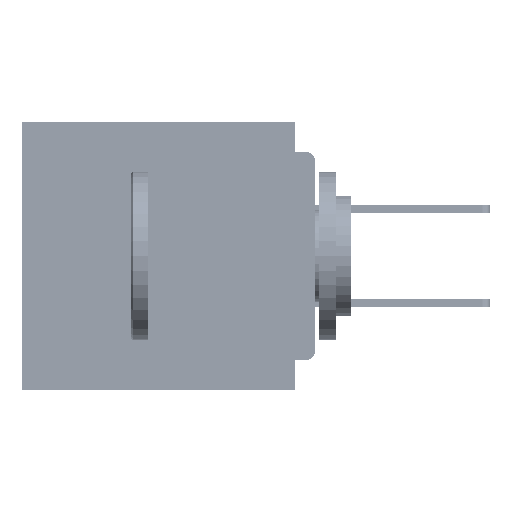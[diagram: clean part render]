
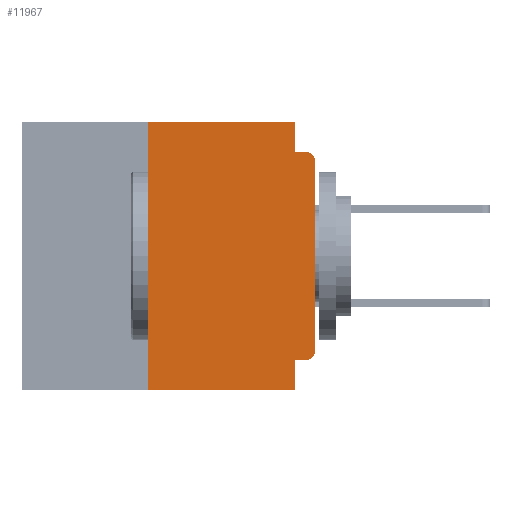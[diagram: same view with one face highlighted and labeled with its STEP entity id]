
A CAD part, left-side view. The second image highlights one B-rep face of the part: STEP entity #11967.
In plain terms, the highlighted planar face has unit normal (-1, 0, 0).
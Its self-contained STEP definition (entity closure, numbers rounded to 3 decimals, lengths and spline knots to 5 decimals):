
#201 = VERTEX_POINT ( 'NONE', #17574 ) ;
#924 = DIRECTION ( 'NONE',  ( 0., 0., -1. ) ) ;
#1513 = EDGE_LOOP ( 'NONE', ( #3939, #25985, #49332, #69862, #61887, #24744, #14929, #63071, #38766, #44028 ) ) ;
#2247 = CARTESIAN_POINT ( 'NONE',  ( 0., 0., -0.045 ) ) ;
#2637 = VERTEX_POINT ( 'NONE', #37194 ) ;
#2857 = CARTESIAN_POINT ( 'NONE',  ( 0., 0.031, -0.4 ) ) ;
#3939 = ORIENTED_EDGE ( 'NONE', *, *, #6980, .T. ) ;
#5364 = DIRECTION ( 'NONE',  ( 0., 0., -1. ) ) ;
#5415 = CARTESIAN_POINT ( 'NONE',  ( 0., 0.437, 0. ) ) ;
#6327 = EDGE_CURVE ( 'NONE', #10774, #26623, #25979, .T. ) ;
#6847 = EDGE_CURVE ( 'NONE', #24629, #201, #35214, .T. ) ;
#6980 = EDGE_CURVE ( 'NONE', #7805, #2637, #14034, .T. ) ;
#7805 = VERTEX_POINT ( 'NONE', #23921 ) ;
#8102 = AXIS2_PLACEMENT_3D ( 'NONE', #65851, #33488, #924 ) ;
#8558 = CIRCLE ( 'NONE', #18196, 0.015 ) ;
#9969 = VECTOR ( 'NONE', #40215, 39.37008 ) ;
#10774 = VERTEX_POINT ( 'NONE', #66708 ) ;
#11110 = VECTOR ( 'NONE', #17274, 39.37008 ) ;
#11600 = VECTOR ( 'NONE', #31241, 39.37008 ) ;
#11956 = AXIS2_PLACEMENT_3D ( 'NONE', #64643, #32281, #70016 ) ;
#11967 = ADVANCED_FACE ( 'NONE', ( #23983 ), #28096, .F. ) ;
#13829 = EDGE_CURVE ( 'NONE', #2637, #44896, #8558, .T. ) ;
#13956 = EDGE_CURVE ( 'NONE', #46617, #201, #25480, .T. ) ;
#14034 = LINE ( 'NONE', #20472, #26718 ) ;
#14929 = ORIENTED_EDGE ( 'NONE', *, *, #13956, .T. ) ;
#15900 = EDGE_CURVE ( 'NONE', #26623, #44896, #38730, .T. ) ;
#17274 = DIRECTION ( 'NONE',  ( 0., -1., 0. ) ) ;
#17574 = CARTESIAN_POINT ( 'NONE',  ( 0., 0.031, -0.4 ) ) ;
#18196 = AXIS2_PLACEMENT_3D ( 'NONE', #70177, #37899, #5364 ) ;
#19271 = LINE ( 'NONE', #5415, #60777 ) ;
#20472 = CARTESIAN_POINT ( 'NONE',  ( 0., 0., 0. ) ) ;
#20813 = VECTOR ( 'NONE', #62591, 39.37008 ) ;
#22179 = LINE ( 'NONE', #56185, #38285 ) ;
#22915 = VERTEX_POINT ( 'NONE', #46774 ) ;
#23921 = CARTESIAN_POINT ( 'NONE',  ( 0., 0., -0.34 ) ) ;
#23983 = FACE_OUTER_BOUND ( 'NONE', #1513, .T. ) ;
#24629 = VERTEX_POINT ( 'NONE', #61502 ) ;
#24744 = ORIENTED_EDGE ( 'NONE', *, *, #57403, .F. ) ;
#25480 = LINE ( 'NONE', #33363, #11110 ) ;
#25766 = CARTESIAN_POINT ( 'NONE',  ( 0., 0.031, 0. ) ) ;
#25979 = LINE ( 'NONE', #25766, #11600 ) ;
#25985 = ORIENTED_EDGE ( 'NONE', *, *, #13829, .T. ) ;
#26623 = VERTEX_POINT ( 'NONE', #43813 ) ;
#26718 = VECTOR ( 'NONE', #58085, 39.37008 ) ;
#28096 = PLANE ( 'NONE',  #8102 ) ;
#30195 = EDGE_CURVE ( 'NONE', #22915, #7805, #56500, .T. ) ;
#31241 = DIRECTION ( 'NONE',  ( 0., 0., -1. ) ) ;
#32281 = DIRECTION ( 'NONE',  ( -1., 0., 0. ) ) ;
#33363 = CARTESIAN_POINT ( 'NONE',  ( 0., 0.437, -0.4 ) ) ;
#33488 = DIRECTION ( 'NONE',  ( 1., 0., 0. ) ) ;
#35214 = LINE ( 'NONE', #2857, #20813 ) ;
#36035 = DIRECTION ( 'NONE',  ( 0., 1., 0. ) ) ;
#37194 = CARTESIAN_POINT ( 'NONE',  ( 0., 0., -0.06 ) ) ;
#37899 = DIRECTION ( 'NONE',  ( -1., 0., 0. ) ) ;
#37954 = DIRECTION ( 'NONE',  ( 0., -1., 0. ) ) ;
#38285 = VECTOR ( 'NONE', #61659, 39.37008 ) ;
#38730 = LINE ( 'NONE', #2247, #9969 ) ;
#38766 = ORIENTED_EDGE ( 'NONE', *, *, #65491, .F. ) ;
#40215 = DIRECTION ( 'NONE',  ( 0., -1., 0. ) ) ;
#43813 = CARTESIAN_POINT ( 'NONE',  ( 0., 0.031, -0.045 ) ) ;
#44028 = ORIENTED_EDGE ( 'NONE', *, *, #30195, .T. ) ;
#44896 = VERTEX_POINT ( 'NONE', #45985 ) ;
#45045 = VECTOR ( 'NONE', #36035, 39.37008 ) ;
#45985 = CARTESIAN_POINT ( 'NONE',  ( 0., 0.015, -0.045 ) ) ;
#46617 = VERTEX_POINT ( 'NONE', #57478 ) ;
#46774 = CARTESIAN_POINT ( 'NONE',  ( 0., 0.015, -0.355 ) ) ;
#49332 = ORIENTED_EDGE ( 'NONE', *, *, #15900, .F. ) ;
#52560 = CARTESIAN_POINT ( 'NONE',  ( 0., 0.25, 0. ) ) ;
#56185 = CARTESIAN_POINT ( 'NONE',  ( 0., 0.25, -0.4 ) ) ;
#56500 = CIRCLE ( 'NONE', #11956, 0.015 ) ;
#57403 = EDGE_CURVE ( 'NONE', #46617, #65519, #22179, .T. ) ;
#57478 = CARTESIAN_POINT ( 'NONE',  ( 0., 0.25, -0.4 ) ) ;
#57531 = CARTESIAN_POINT ( 'NONE',  ( 0., 0., -0.355 ) ) ;
#58085 = DIRECTION ( 'NONE',  ( 0., 0., 1. ) ) ;
#59482 = LINE ( 'NONE', #57531, #45045 ) ;
#60777 = VECTOR ( 'NONE', #37954, 39.37008 ) ;
#61502 = CARTESIAN_POINT ( 'NONE',  ( 0., 0.031, -0.355 ) ) ;
#61659 = DIRECTION ( 'NONE',  ( 0., 0., 1. ) ) ;
#61887 = ORIENTED_EDGE ( 'NONE', *, *, #66527, .F. ) ;
#62591 = DIRECTION ( 'NONE',  ( 0., 0., -1. ) ) ;
#63071 = ORIENTED_EDGE ( 'NONE', *, *, #6847, .F. ) ;
#64643 = CARTESIAN_POINT ( 'NONE',  ( 0., 0.015, -0.34 ) ) ;
#65491 = EDGE_CURVE ( 'NONE', #22915, #24629, #59482, .T. ) ;
#65519 = VERTEX_POINT ( 'NONE', #52560 ) ;
#65851 = CARTESIAN_POINT ( 'NONE',  ( 0., 0.437, 0. ) ) ;
#66527 = EDGE_CURVE ( 'NONE', #65519, #10774, #19271, .T. ) ;
#66708 = CARTESIAN_POINT ( 'NONE',  ( 0., 0.031, 0. ) ) ;
#69862 = ORIENTED_EDGE ( 'NONE', *, *, #6327, .F. ) ;
#70016 = DIRECTION ( 'NONE',  ( 0., 0., -1. ) ) ;
#70177 = CARTESIAN_POINT ( 'NONE',  ( 0., 0.015, -0.06 ) ) ;
